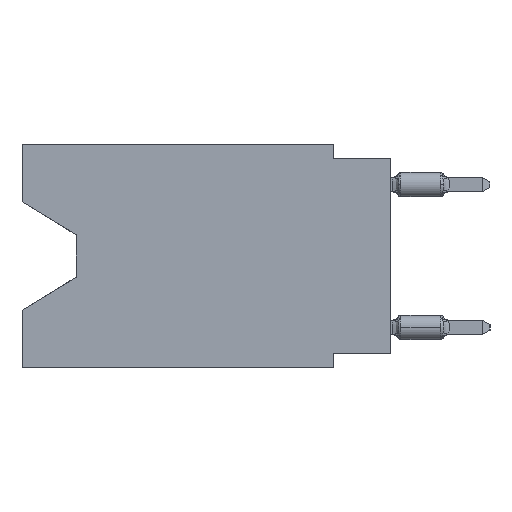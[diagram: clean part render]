
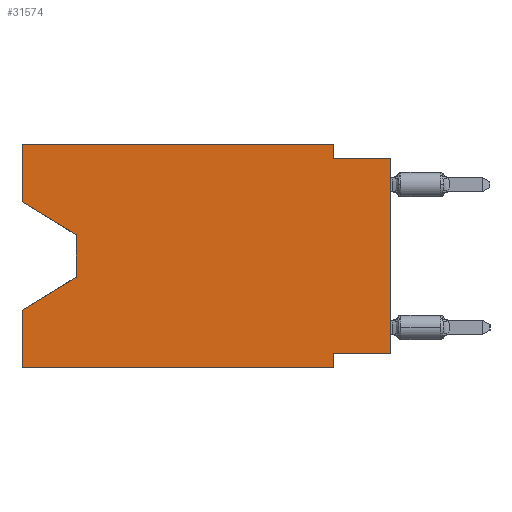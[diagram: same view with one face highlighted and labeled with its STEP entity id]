
A CAD part, left-side view. The second image highlights one B-rep face of the part: STEP entity #31574.
In plain terms, the highlighted planar face has unit normal (-1, 0, 0).
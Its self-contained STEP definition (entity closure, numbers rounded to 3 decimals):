
#680 = DIRECTION ( 'NONE',  ( 0., 0., -1. ) ) ;
#1622 = LINE ( 'NONE', #57813, #61613 ) ;
#2162 = CARTESIAN_POINT ( 'NONE',  ( 0., 2.54, -9.271 ) ) ;
#2252 = DIRECTION ( 'NONE',  ( 0., 0., -1. ) ) ;
#2330 = EDGE_CURVE ( 'NONE', #60118, #34629, #18297, .T. ) ;
#2456 = DIRECTION ( 'NONE',  ( 0., 0., -1. ) ) ;
#2698 = VECTOR ( 'NONE', #6367, 1000. ) ;
#3260 = VERTEX_POINT ( 'NONE', #33178 ) ;
#3459 = VERTEX_POINT ( 'NONE', #21846 ) ;
#3525 = EDGE_CURVE ( 'NONE', #15602, #10732, #51978, .T. ) ;
#3626 = CARTESIAN_POINT ( 'NONE',  ( 0., 13.97, -4.013 ) ) ;
#4800 = CARTESIAN_POINT ( 'NONE',  ( 0., 0., -0.635 ) ) ;
#5936 = CARTESIAN_POINT ( 'NONE',  ( 0., 0., -9.271 ) ) ;
#6367 = DIRECTION ( 'NONE',  ( 0., 0., 1. ) ) ;
#6525 = CARTESIAN_POINT ( 'NONE',  ( 0., 16.383, 0. ) ) ;
#7663 = ORIENTED_EDGE ( 'NONE', *, *, #12668, .F. ) ;
#8061 = ORIENTED_EDGE ( 'NONE', *, *, #20165, .F. ) ;
#8192 = ORIENTED_EDGE ( 'NONE', *, *, #37525, .T. ) ;
#8862 = CARTESIAN_POINT ( 'NONE',  ( 0., 2.54, -0.635 ) ) ;
#9082 = CARTESIAN_POINT ( 'NONE',  ( 0., 16.383, 0. ) ) ;
#10281 = DIRECTION ( 'NONE',  ( 0., -1., 0. ) ) ;
#10732 = VERTEX_POINT ( 'NONE', #3626 ) ;
#10784 = VECTOR ( 'NONE', #25330, 1000. ) ;
#11452 = EDGE_CURVE ( 'NONE', #59871, #35255, #1622, .T. ) ;
#11477 = DIRECTION ( 'NONE',  ( 0., 0., -1. ) ) ;
#11560 = PLANE ( 'NONE',  #46805 ) ;
#11699 = CARTESIAN_POINT ( 'NONE',  ( 0., 0., -0.635 ) ) ;
#11999 = CARTESIAN_POINT ( 'NONE',  ( 0., 0., 0. ) ) ;
#12668 = EDGE_CURVE ( 'NONE', #35255, #31840, #50005, .T. ) ;
#12763 = VECTOR ( 'NONE', #42215, 1000. ) ;
#15602 = VERTEX_POINT ( 'NONE', #27921 ) ;
#16198 = EDGE_CURVE ( 'NONE', #10732, #3459, #60420, .T. ) ;
#17105 = CARTESIAN_POINT ( 'NONE',  ( 0., 13.97, -4.013 ) ) ;
#18297 = LINE ( 'NONE', #37429, #48868 ) ;
#19963 = VECTOR ( 'NONE', #40253, 1000. ) ;
#20165 = EDGE_CURVE ( 'NONE', #3260, #21549, #24433, .T. ) ;
#20814 = LINE ( 'NONE', #35240, #19963 ) ;
#21329 = CARTESIAN_POINT ( 'NONE',  ( 0., 16.383, -7.36 ) ) ;
#21549 = VERTEX_POINT ( 'NONE', #2162 ) ;
#21846 = CARTESIAN_POINT ( 'NONE',  ( 0., 13.97, -5.893 ) ) ;
#21938 = CARTESIAN_POINT ( 'NONE',  ( 0., 2.54, 0. ) ) ;
#22482 = VECTOR ( 'NONE', #61923, 1000. ) ;
#22782 = EDGE_CURVE ( 'NONE', #21549, #34629, #49970, .T. ) ;
#23617 = LINE ( 'NONE', #38051, #22482 ) ;
#23725 = EDGE_LOOP ( 'NONE', ( #61160, #60203, #8192, #35043, #42235, #28285, #8061, #34306, #7663, #40728, #53002, #27220 ) ) ;
#24433 = LINE ( 'NONE', #5936, #28202 ) ;
#25051 = DIRECTION ( 'NONE',  ( 0., 1., 0. ) ) ;
#25330 = DIRECTION ( 'NONE',  ( 0., 0.855, -0.519 ) ) ;
#27220 = ORIENTED_EDGE ( 'NONE', *, *, #41185, .F. ) ;
#27921 = CARTESIAN_POINT ( 'NONE',  ( 0., 16.383, -2.546 ) ) ;
#28202 = VECTOR ( 'NONE', #25051, 1000. ) ;
#28285 = ORIENTED_EDGE ( 'NONE', *, *, #22782, .F. ) ;
#30356 = FACE_OUTER_BOUND ( 'NONE', #23725, .T. ) ;
#31092 = CARTESIAN_POINT ( 'NONE',  ( 0., 2.54, -9.906 ) ) ;
#31574 = ADVANCED_FACE ( 'NONE', ( #30356 ), #11560, .F. ) ;
#31840 = VERTEX_POINT ( 'NONE', #4800 ) ;
#32522 = VERTEX_POINT ( 'NONE', #21329 ) ;
#32714 = DIRECTION ( 'NONE',  ( 0., -1., 0. ) ) ;
#33178 = CARTESIAN_POINT ( 'NONE',  ( 0., 0., -9.271 ) ) ;
#34306 = ORIENTED_EDGE ( 'NONE', *, *, #36677, .T. ) ;
#34629 = VERTEX_POINT ( 'NONE', #40635 ) ;
#34640 = VECTOR ( 'NONE', #56489, 1000. ) ;
#35043 = ORIENTED_EDGE ( 'NONE', *, *, #47240, .F. ) ;
#35240 = CARTESIAN_POINT ( 'NONE',  ( 0., 16.383, 0. ) ) ;
#35255 = VERTEX_POINT ( 'NONE', #8862 ) ;
#36677 = EDGE_CURVE ( 'NONE', #3260, #31840, #54062, .T. ) ;
#37429 = CARTESIAN_POINT ( 'NONE',  ( 0., 16.383, -9.906 ) ) ;
#37525 = EDGE_CURVE ( 'NONE', #3459, #32522, #49200, .T. ) ;
#38051 = CARTESIAN_POINT ( 'NONE',  ( 0., 16.383, 0. ) ) ;
#38917 = VECTOR ( 'NONE', #11477, 1000. ) ;
#39134 = VECTOR ( 'NONE', #10281, 1000. ) ;
#39432 = LINE ( 'NONE', #6525, #39134 ) ;
#40253 = DIRECTION ( 'NONE',  ( 0., 0., 1. ) ) ;
#40635 = CARTESIAN_POINT ( 'NONE',  ( 0., 2.54, -9.906 ) ) ;
#40728 = ORIENTED_EDGE ( 'NONE', *, *, #11452, .F. ) ;
#41185 = EDGE_CURVE ( 'NONE', #15602, #55144, #20814, .T. ) ;
#42215 = DIRECTION ( 'NONE',  ( 0., -0.855, -0.519 ) ) ;
#42235 = ORIENTED_EDGE ( 'NONE', *, *, #2330, .T. ) ;
#45124 = CARTESIAN_POINT ( 'NONE',  ( 0., 16.383, 0. ) ) ;
#46429 = VECTOR ( 'NONE', #2252, 1000. ) ;
#46805 = AXIS2_PLACEMENT_3D ( 'NONE', #45124, #49547, #2456 ) ;
#47240 = EDGE_CURVE ( 'NONE', #60118, #32522, #23617, .T. ) ;
#48868 = VECTOR ( 'NONE', #32714, 1000. ) ;
#49200 = LINE ( 'NONE', #54225, #10784 ) ;
#49448 = EDGE_CURVE ( 'NONE', #55144, #59871, #39432, .T. ) ;
#49547 = DIRECTION ( 'NONE',  ( 1., 0., 0. ) ) ;
#49970 = LINE ( 'NONE', #31092, #46429 ) ;
#50005 = LINE ( 'NONE', #11699, #34640 ) ;
#51978 = LINE ( 'NONE', #55757, #12763 ) ;
#53002 = ORIENTED_EDGE ( 'NONE', *, *, #49448, .F. ) ;
#53601 = CARTESIAN_POINT ( 'NONE',  ( 0., 16.383, -9.906 ) ) ;
#54062 = LINE ( 'NONE', #11999, #2698 ) ;
#54225 = CARTESIAN_POINT ( 'NONE',  ( 0., 13.97, -5.893 ) ) ;
#55144 = VERTEX_POINT ( 'NONE', #9082 ) ;
#55757 = CARTESIAN_POINT ( 'NONE',  ( 0., 16.383, -2.546 ) ) ;
#56489 = DIRECTION ( 'NONE',  ( 0., -1., 0. ) ) ;
#57813 = CARTESIAN_POINT ( 'NONE',  ( 0., 2.54, 0. ) ) ;
#59871 = VERTEX_POINT ( 'NONE', #21938 ) ;
#60118 = VERTEX_POINT ( 'NONE', #53601 ) ;
#60203 = ORIENTED_EDGE ( 'NONE', *, *, #16198, .T. ) ;
#60420 = LINE ( 'NONE', #17105, #38917 ) ;
#61160 = ORIENTED_EDGE ( 'NONE', *, *, #3525, .T. ) ;
#61613 = VECTOR ( 'NONE', #680, 1000. ) ;
#61923 = DIRECTION ( 'NONE',  ( 0., 0., 1. ) ) ;
